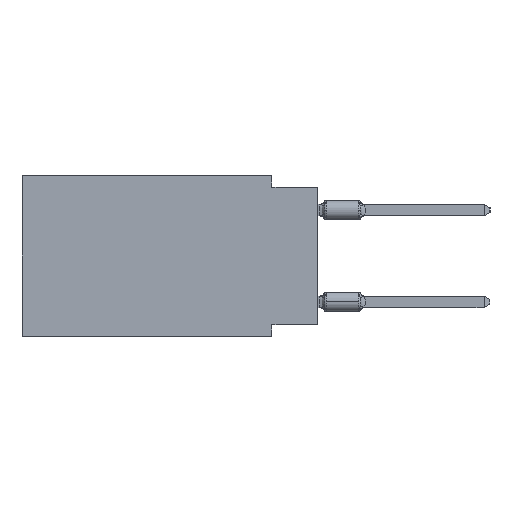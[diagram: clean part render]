
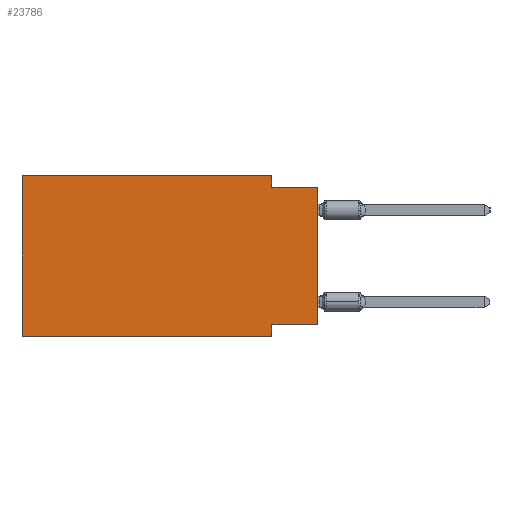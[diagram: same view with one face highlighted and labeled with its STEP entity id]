
A CAD part, left-side view. The second image highlights one B-rep face of the part: STEP entity #23786.
In plain terms, the highlighted planar face has unit normal (-1, 0, 0).
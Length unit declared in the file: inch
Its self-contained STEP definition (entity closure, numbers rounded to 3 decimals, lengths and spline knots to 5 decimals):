
#1109 = EDGE_CURVE ( 'NONE', #11012, #26254, #14478, .T. ) ;
#1612 = EDGE_CURVE ( 'NONE', #24839, #5278, #7366, .T. ) ;
#2233 = DIRECTION ( 'NONE',  ( 1., 0., 0. ) ) ;
#2251 = CARTESIAN_POINT ( 'NONE',  ( 0., 0.645, 0. ) ) ;
#2367 = DIRECTION ( 'NONE',  ( 0., 0., -1. ) ) ;
#2659 = DIRECTION ( 'NONE',  ( 0., 0., -1. ) ) ;
#3060 = LINE ( 'NONE', #6670, #21578 ) ;
#3203 = VECTOR ( 'NONE', #2659, 39.37008 ) ;
#3386 = LINE ( 'NONE', #13591, #11970 ) ;
#3614 = VECTOR ( 'NONE', #12632, 39.37008 ) ;
#3834 = EDGE_CURVE ( 'NONE', #11012, #25251, #22321, .T. ) ;
#4704 = VERTEX_POINT ( 'NONE', #13724 ) ;
#4862 = VECTOR ( 'NONE', #22451, 39.37008 ) ;
#4905 = LINE ( 'NONE', #17002, #3203 ) ;
#5278 = VERTEX_POINT ( 'NONE', #10790 ) ;
#5301 = CARTESIAN_POINT ( 'NONE',  ( 0., 0.1, 0. ) ) ;
#6104 = CARTESIAN_POINT ( 'NONE',  ( 0., 0., -0.325 ) ) ;
#6132 = EDGE_CURVE ( 'NONE', #24276, #26254, #10333, .T. ) ;
#6317 = EDGE_CURVE ( 'NONE', #12457, #4704, #4905, .T. ) ;
#6670 = CARTESIAN_POINT ( 'NONE',  ( 0., 0.645, 0. ) ) ;
#7236 = DIRECTION ( 'NONE',  ( 0., 1., 0. ) ) ;
#7366 = LINE ( 'NONE', #11601, #18949 ) ;
#7848 = EDGE_CURVE ( 'NONE', #4704, #5278, #14561, .T. ) ;
#8055 = CARTESIAN_POINT ( 'NONE',  ( 0., 0.645, 0. ) ) ;
#10333 = LINE ( 'NONE', #18452, #19747 ) ;
#10652 = CARTESIAN_POINT ( 'NONE',  ( 0., 0.645, -0.35 ) ) ;
#10790 = CARTESIAN_POINT ( 'NONE',  ( 0., 0., -0.025 ) ) ;
#11012 = VERTEX_POINT ( 'NONE', #16399 ) ;
#11106 = AXIS2_PLACEMENT_3D ( 'NONE', #16295, #2233, #22437 ) ;
#11149 = ORIENTED_EDGE ( 'NONE', *, *, #6317, .F. ) ;
#11601 = CARTESIAN_POINT ( 'NONE',  ( 0., 0., 0. ) ) ;
#11970 = VECTOR ( 'NONE', #7236, 39.37008 ) ;
#12457 = VERTEX_POINT ( 'NONE', #5301 ) ;
#12632 = DIRECTION ( 'NONE',  ( 0., -1., 0. ) ) ;
#13591 = CARTESIAN_POINT ( 'NONE',  ( 0., 0., -0.325 ) ) ;
#13724 = CARTESIAN_POINT ( 'NONE',  ( 0., 0.1, -0.025 ) ) ;
#14302 = CARTESIAN_POINT ( 'NONE',  ( 0., 0., -0.025 ) ) ;
#14478 = LINE ( 'NONE', #10652, #3614 ) ;
#14561 = LINE ( 'NONE', #14302, #15918 ) ;
#14860 = DIRECTION ( 'NONE',  ( 0., -1., 0. ) ) ;
#15735 = ORIENTED_EDGE ( 'NONE', *, *, #1109, .T. ) ;
#15918 = VECTOR ( 'NONE', #18326, 39.37008 ) ;
#16295 = CARTESIAN_POINT ( 'NONE',  ( 0., 0.645, 0. ) ) ;
#16399 = CARTESIAN_POINT ( 'NONE',  ( 0., 0.645, -0.35 ) ) ;
#17002 = CARTESIAN_POINT ( 'NONE',  ( 0., 0.1, 0. ) ) ;
#17249 = ORIENTED_EDGE ( 'NONE', *, *, #7848, .F. ) ;
#17686 = EDGE_CURVE ( 'NONE', #25251, #12457, #3060, .T. ) ;
#18326 = DIRECTION ( 'NONE',  ( 0., -1., 0. ) ) ;
#18408 = ORIENTED_EDGE ( 'NONE', *, *, #6132, .F. ) ;
#18452 = CARTESIAN_POINT ( 'NONE',  ( 0., 0.1, -0.35 ) ) ;
#18949 = VECTOR ( 'NONE', #19601, 39.37008 ) ;
#19601 = DIRECTION ( 'NONE',  ( 0., 0., 1. ) ) ;
#19747 = VECTOR ( 'NONE', #2367, 39.37008 ) ;
#20840 = FACE_OUTER_BOUND ( 'NONE', #23106, .T. ) ;
#21318 = ORIENTED_EDGE ( 'NONE', *, *, #3834, .F. ) ;
#21578 = VECTOR ( 'NONE', #14860, 39.37008 ) ;
#21752 = ORIENTED_EDGE ( 'NONE', *, *, #17686, .F. ) ;
#22321 = LINE ( 'NONE', #2251, #4862 ) ;
#22437 = DIRECTION ( 'NONE',  ( 0., 0., -1. ) ) ;
#22451 = DIRECTION ( 'NONE',  ( 0., 0., 1. ) ) ;
#23106 = EDGE_LOOP ( 'NONE', ( #26118, #17249, #11149, #21752, #21318, #15735, #18408, #25092 ) ) ;
#23786 = ADVANCED_FACE ( 'NONE', ( #20840 ), #26277, .F. ) ;
#23900 = CARTESIAN_POINT ( 'NONE',  ( 0., 0.1, -0.35 ) ) ;
#24276 = VERTEX_POINT ( 'NONE', #25578 ) ;
#24312 = EDGE_CURVE ( 'NONE', #24839, #24276, #3386, .T. ) ;
#24839 = VERTEX_POINT ( 'NONE', #6104 ) ;
#25092 = ORIENTED_EDGE ( 'NONE', *, *, #24312, .F. ) ;
#25251 = VERTEX_POINT ( 'NONE', #8055 ) ;
#25578 = CARTESIAN_POINT ( 'NONE',  ( 0., 0.1, -0.325 ) ) ;
#26118 = ORIENTED_EDGE ( 'NONE', *, *, #1612, .T. ) ;
#26254 = VERTEX_POINT ( 'NONE', #23900 ) ;
#26277 = PLANE ( 'NONE',  #11106 ) ;
